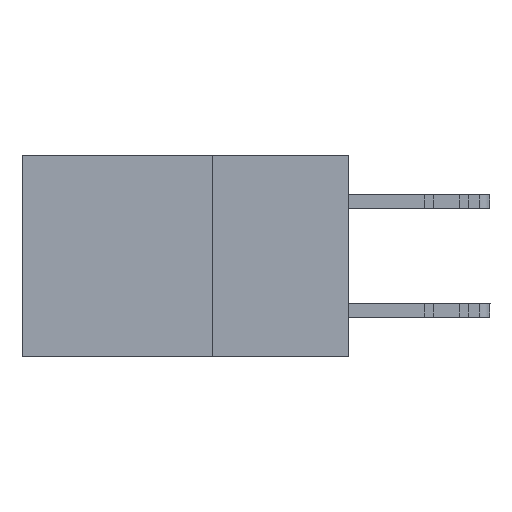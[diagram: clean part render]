
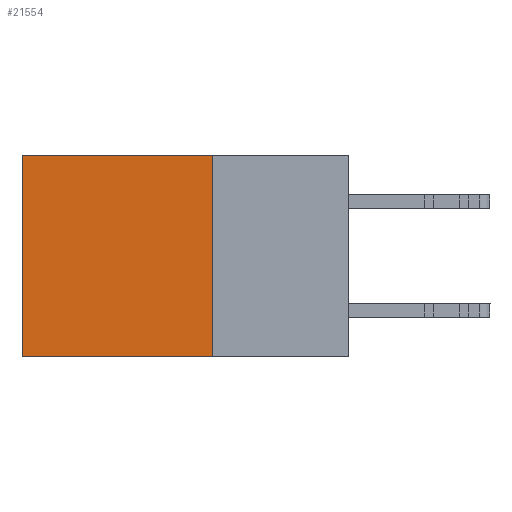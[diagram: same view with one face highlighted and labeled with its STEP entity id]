
A CAD part, left-side view. The second image highlights one B-rep face of the part: STEP entity #21554.
In plain terms, the highlighted planar face has unit normal (-1, 0, 0).
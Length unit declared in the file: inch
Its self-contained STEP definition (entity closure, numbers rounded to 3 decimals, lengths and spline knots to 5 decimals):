
#979 = VECTOR ( 'NONE', #8638, 39.37008 ) ;
#2154 = ORIENTED_EDGE ( 'NONE', *, *, #23048, .T. ) ;
#2560 = LINE ( 'NONE', #18832, #979 ) ;
#2916 = ORIENTED_EDGE ( 'NONE', *, *, #19061, .T. ) ;
#4396 = EDGE_CURVE ( 'NONE', #12154, #26171, #2560, .T. ) ;
#5149 = DIRECTION ( 'NONE',  ( 0., 0., -1. ) ) ;
#5830 = CARTESIAN_POINT ( 'NONE',  ( 0.298, 0.6, 0. ) ) ;
#7617 = CARTESIAN_POINT ( 'NONE',  ( 0.298, 0.25, 0. ) ) ;
#7747 = FACE_OUTER_BOUND ( 'NONE', #10344, .T. ) ;
#8318 = ORIENTED_EDGE ( 'NONE', *, *, #32192, .F. ) ;
#8638 = DIRECTION ( 'NONE',  ( 0., 1., 0. ) ) ;
#10344 = EDGE_LOOP ( 'NONE', ( #2916, #32253, #8318, #2154 ) ) ;
#11370 = DIRECTION ( 'NONE',  ( 1., 0., 0. ) ) ;
#11435 = LINE ( 'NONE', #5830, #12595 ) ;
#12154 = VERTEX_POINT ( 'NONE', #14665 ) ;
#12595 = VECTOR ( 'NONE', #21100, 39.37008 ) ;
#12908 = LINE ( 'NONE', #30463, #32143 ) ;
#14665 = CARTESIAN_POINT ( 'NONE',  ( 0.298, 0.25, -0.37 ) ) ;
#15110 = VERTEX_POINT ( 'NONE', #30289 ) ;
#16293 = DIRECTION ( 'NONE',  ( 0., 0., -1. ) ) ;
#18706 = PLANE ( 'NONE',  #22941 ) ;
#18832 = CARTESIAN_POINT ( 'NONE',  ( 0.298, 0.25, -0.37 ) ) ;
#19025 = VERTEX_POINT ( 'NONE', #20992 ) ;
#19061 = EDGE_CURVE ( 'NONE', #15110, #26171, #11435, .T. ) ;
#20992 = CARTESIAN_POINT ( 'NONE',  ( 0.298, 0.25, 0. ) ) ;
#21028 = VECTOR ( 'NONE', #25162, 39.37008 ) ;
#21100 = DIRECTION ( 'NONE',  ( 0., 0., -1. ) ) ;
#21259 = CARTESIAN_POINT ( 'NONE',  ( 0.298, 0.25, 0. ) ) ;
#21554 = ADVANCED_FACE ( 'NONE', ( #7747 ), #18706, .F. ) ;
#22941 = AXIS2_PLACEMENT_3D ( 'NONE', #21259, #11370, #16293 ) ;
#23048 = EDGE_CURVE ( 'NONE', #19025, #15110, #27664, .T. ) ;
#25162 = DIRECTION ( 'NONE',  ( 0., 1., 0. ) ) ;
#26171 = VERTEX_POINT ( 'NONE', #29700 ) ;
#27664 = LINE ( 'NONE', #7617, #21028 ) ;
#29700 = CARTESIAN_POINT ( 'NONE',  ( 0.298, 0.6, -0.37 ) ) ;
#30289 = CARTESIAN_POINT ( 'NONE',  ( 0.298, 0.6, 0. ) ) ;
#30463 = CARTESIAN_POINT ( 'NONE',  ( 0.298, 0.25, 0. ) ) ;
#32143 = VECTOR ( 'NONE', #5149, 39.37008 ) ;
#32192 = EDGE_CURVE ( 'NONE', #19025, #12154, #12908, .T. ) ;
#32253 = ORIENTED_EDGE ( 'NONE', *, *, #4396, .F. ) ;
